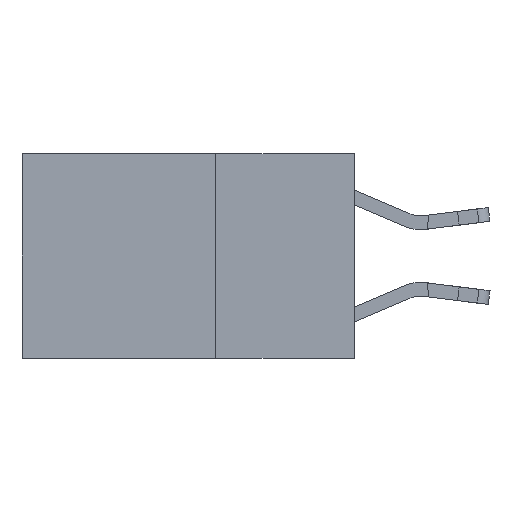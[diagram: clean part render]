
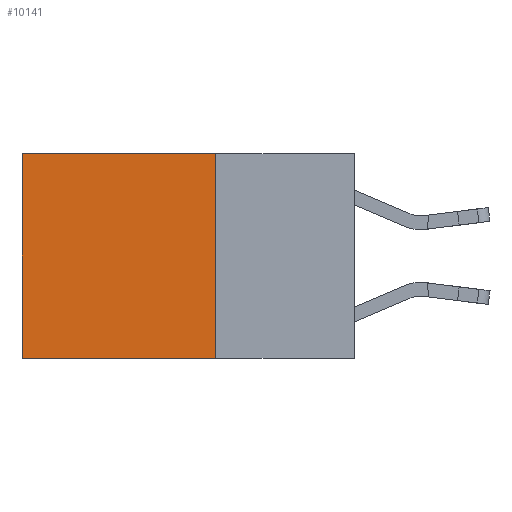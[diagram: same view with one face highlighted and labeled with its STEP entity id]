
A CAD part, left-side view. The second image highlights one B-rep face of the part: STEP entity #10141.
In plain terms, the highlighted planar face has unit normal (-1, 0, 0).
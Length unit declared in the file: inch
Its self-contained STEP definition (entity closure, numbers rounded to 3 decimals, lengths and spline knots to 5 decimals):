
#250 = EDGE_CURVE ( 'NONE', #11660, #2171, #1665, .T. ) ;
#436 = EDGE_CURVE ( 'NONE', #2336, #717, #4677, .T. ) ;
#665 = CARTESIAN_POINT ( 'NONE',  ( 0.2625, 0.25, -0.37 ) ) ;
#690 = ORIENTED_EDGE ( 'NONE', *, *, #250, .T. ) ;
#717 = VERTEX_POINT ( 'NONE', #665 ) ;
#843 = CARTESIAN_POINT ( 'NONE',  ( 0.2625, 0.6, -0.37 ) ) ;
#1115 = EDGE_LOOP ( 'NONE', ( #690, #10932, #14000, #7038 ) ) ;
#1315 = VECTOR ( 'NONE', #4673, 39.37008 ) ;
#1665 = LINE ( 'NONE', #2233, #1315 ) ;
#2171 = VERTEX_POINT ( 'NONE', #843 ) ;
#2178 = FACE_OUTER_BOUND ( 'NONE', #1115, .T. ) ;
#2233 = CARTESIAN_POINT ( 'NONE',  ( 0.2625, 0.6, 0. ) ) ;
#2336 = VERTEX_POINT ( 'NONE', #10600 ) ;
#3576 = DIRECTION ( 'NONE',  ( 0., 1., 0. ) ) ;
#3745 = VECTOR ( 'NONE', #6736, 39.37008 ) ;
#4489 = LINE ( 'NONE', #6644, #3745 ) ;
#4673 = DIRECTION ( 'NONE',  ( 0., 0., -1. ) ) ;
#4677 = LINE ( 'NONE', #9649, #9562 ) ;
#4691 = CARTESIAN_POINT ( 'NONE',  ( 0.2625, 0.6, 0. ) ) ;
#4879 = DIRECTION ( 'NONE',  ( 0., 0., -1. ) ) ;
#4915 = LINE ( 'NONE', #12537, #11900 ) ;
#6324 = EDGE_CURVE ( 'NONE', #2336, #11660, #4489, .T. ) ;
#6644 = CARTESIAN_POINT ( 'NONE',  ( 0.2625, 0.25, 0. ) ) ;
#6736 = DIRECTION ( 'NONE',  ( 0., 1., 0. ) ) ;
#7038 = ORIENTED_EDGE ( 'NONE', *, *, #6324, .T. ) ;
#7262 = DIRECTION ( 'NONE',  ( 1., 0., 0. ) ) ;
#7592 = DIRECTION ( 'NONE',  ( 0., 0., -1. ) ) ;
#9453 = AXIS2_PLACEMENT_3D ( 'NONE', #13932, #7262, #4879 ) ;
#9562 = VECTOR ( 'NONE', #7592, 39.37008 ) ;
#9649 = CARTESIAN_POINT ( 'NONE',  ( 0.2625, 0.25, 0. ) ) ;
#10141 = ADVANCED_FACE ( 'NONE', ( #2178 ), #10555, .F. ) ;
#10555 = PLANE ( 'NONE',  #9453 ) ;
#10600 = CARTESIAN_POINT ( 'NONE',  ( 0.2625, 0.25, 0. ) ) ;
#10932 = ORIENTED_EDGE ( 'NONE', *, *, #13407, .F. ) ;
#11660 = VERTEX_POINT ( 'NONE', #4691 ) ;
#11900 = VECTOR ( 'NONE', #3576, 39.37008 ) ;
#12537 = CARTESIAN_POINT ( 'NONE',  ( 0.2625, 0.25, -0.37 ) ) ;
#13407 = EDGE_CURVE ( 'NONE', #717, #2171, #4915, .T. ) ;
#13932 = CARTESIAN_POINT ( 'NONE',  ( 0.2625, 0.25, 0. ) ) ;
#14000 = ORIENTED_EDGE ( 'NONE', *, *, #436, .F. ) ;
